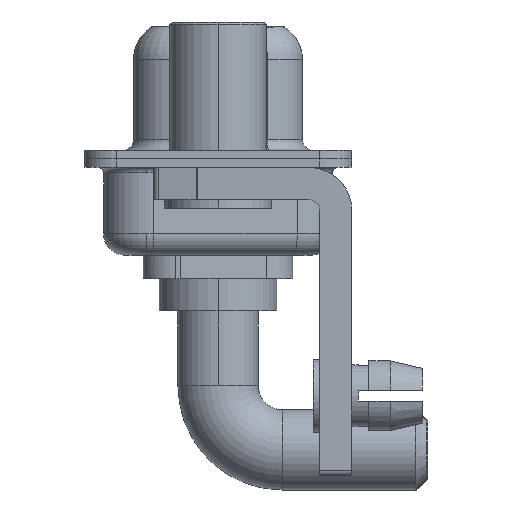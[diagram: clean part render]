
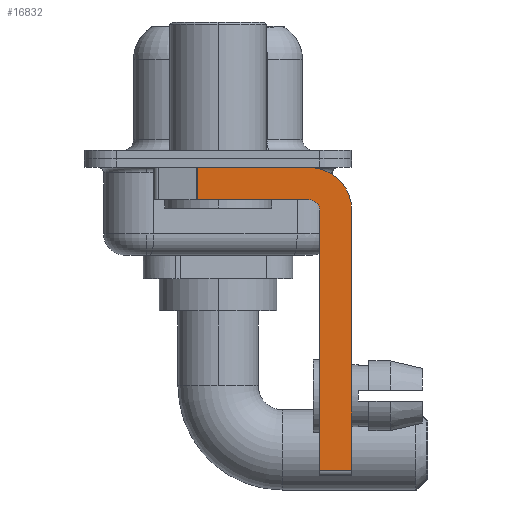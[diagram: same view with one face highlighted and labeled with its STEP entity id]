
A CAD part, left-side view. The second image highlights one B-rep face of the part: STEP entity #16832.
In plain terms, the highlighted planar face has unit normal (-1, 0, 0).
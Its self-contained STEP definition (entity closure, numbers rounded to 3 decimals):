
#1 = CARTESIAN_POINT ( 'NONE',  ( -2.9, -4.25, -1.9 ) ) ;
#162 = DIRECTION ( 'NONE',  ( 1., 0., 0. ) ) ;
#366 = AXIS2_PLACEMENT_3D ( 'NONE', #9549, #162, #2883 ) ;
#743 = ORIENTED_EDGE ( 'NONE', *, *, #10073, .F. ) ;
#809 = AXIS2_PLACEMENT_3D ( 'NONE', #10354, #12896, #15712 ) ;
#1100 = DIRECTION ( 'NONE',  ( 0., -1., 0. ) ) ;
#1345 = CARTESIAN_POINT ( 'NONE',  ( -2.9, 0.978, -1.9 ) ) ;
#1350 = VERTEX_POINT ( 'NONE', #8214 ) ;
#1498 = CARTESIAN_POINT ( 'NONE',  ( -2.9, -4.75, -14.55 ) ) ;
#1647 = ORIENTED_EDGE ( 'NONE', *, *, #7252, .F. ) ;
#1827 = PLANE ( 'NONE',  #366 ) ;
#1841 = DIRECTION ( 'NONE',  ( 0., 0., 1. ) ) ;
#2256 = DIRECTION ( 'NONE',  ( 0., 0., -1. ) ) ;
#2346 = EDGE_CURVE ( 'NONE', #8330, #3171, #4071, .T. ) ;
#2705 = CARTESIAN_POINT ( 'NONE',  ( -2.9, -6.25, -2.4 ) ) ;
#2883 = DIRECTION ( 'NONE',  ( 0., 0., -1. ) ) ;
#2997 = CARTESIAN_POINT ( 'NONE',  ( -2.9, -4.75, -2.4 ) ) ;
#3171 = VERTEX_POINT ( 'NONE', #12413 ) ;
#3783 = LINE ( 'NONE', #11503, #14538 ) ;
#4048 = CARTESIAN_POINT ( 'NONE',  ( -2.9, -6.25, -14.55 ) ) ;
#4071 = LINE ( 'NONE', #1345, #7500 ) ;
#4145 = VECTOR ( 'NONE', #15339, 1000. ) ;
#4991 = DIRECTION ( 'NONE',  ( 0., 0., 1. ) ) ;
#5455 = CIRCLE ( 'NONE', #7958, 0.5 ) ;
#5770 = CARTESIAN_POINT ( 'NONE',  ( -2.9, -4.75, -14.8 ) ) ;
#6132 = CIRCLE ( 'NONE', #809, 2. ) ;
#6222 = EDGE_CURVE ( 'NONE', #14532, #13422, #5455, .T. ) ;
#6990 = EDGE_LOOP ( 'NONE', ( #12298, #10099, #743, #17229, #1647, #15953, #10006, #7535 ) ) ;
#7252 = EDGE_CURVE ( 'NONE', #14864, #14532, #8662, .T. ) ;
#7500 = VECTOR ( 'NONE', #12145, 1000. ) ;
#7535 = ORIENTED_EDGE ( 'NONE', *, *, #10084, .F. ) ;
#7752 = LINE ( 'NONE', #11632, #12132 ) ;
#7958 = AXIS2_PLACEMENT_3D ( 'NONE', #11650, #16993, #4991 ) ;
#8214 = CARTESIAN_POINT ( 'NONE',  ( -2.9, -4.25, -0.4 ) ) ;
#8330 = VERTEX_POINT ( 'NONE', #16807 ) ;
#8662 = LINE ( 'NONE', #5770, #15976 ) ;
#9024 = LINE ( 'NONE', #14377, #4145 ) ;
#9549 = CARTESIAN_POINT ( 'NONE',  ( -2.9, -4.25, -2.4 ) ) ;
#10006 = ORIENTED_EDGE ( 'NONE', *, *, #15042, .F. ) ;
#10073 = EDGE_CURVE ( 'NONE', #13422, #3171, #3783, .T. ) ;
#10084 = EDGE_CURVE ( 'NONE', #1350, #16722, #6132, .T. ) ;
#10099 = ORIENTED_EDGE ( 'NONE', *, *, #2346, .T. ) ;
#10142 = VERTEX_POINT ( 'NONE', #4048 ) ;
#10262 = DIRECTION ( 'NONE',  ( 0., 1., 0. ) ) ;
#10354 = CARTESIAN_POINT ( 'NONE',  ( -2.9, -4.25, -2.4 ) ) ;
#10576 = EDGE_CURVE ( 'NONE', #8330, #1350, #9024, .T. ) ;
#11503 = CARTESIAN_POINT ( 'NONE',  ( -2.9, -4.25, -1.9 ) ) ;
#11632 = CARTESIAN_POINT ( 'NONE',  ( -2.9, -6.25, -2.4 ) ) ;
#11650 = CARTESIAN_POINT ( 'NONE',  ( -2.9, -4.25, -2.4 ) ) ;
#12132 = VECTOR ( 'NONE', #2256, 1000. ) ;
#12145 = DIRECTION ( 'NONE',  ( 0., 0., -1. ) ) ;
#12298 = ORIENTED_EDGE ( 'NONE', *, *, #10576, .F. ) ;
#12413 = CARTESIAN_POINT ( 'NONE',  ( -2.9, 0.978, -1.9 ) ) ;
#12896 = DIRECTION ( 'NONE',  ( 1., 0., 0. ) ) ;
#13422 = VERTEX_POINT ( 'NONE', #1 ) ;
#13781 = VECTOR ( 'NONE', #1100, 1000. ) ;
#14377 = CARTESIAN_POINT ( 'NONE',  ( -2.9, 3., -0.4 ) ) ;
#14436 = LINE ( 'NONE', #17059, #13781 ) ;
#14532 = VERTEX_POINT ( 'NONE', #2997 ) ;
#14538 = VECTOR ( 'NONE', #10262, 1000. ) ;
#14864 = VERTEX_POINT ( 'NONE', #1498 ) ;
#14980 = FACE_OUTER_BOUND ( 'NONE', #6990, .T. ) ;
#15042 = EDGE_CURVE ( 'NONE', #16722, #10142, #7752, .T. ) ;
#15104 = EDGE_CURVE ( 'NONE', #14864, #10142, #14436, .T. ) ;
#15339 = DIRECTION ( 'NONE',  ( 0., -1., 0. ) ) ;
#15712 = DIRECTION ( 'NONE',  ( 0., 0., -1. ) ) ;
#15953 = ORIENTED_EDGE ( 'NONE', *, *, #15104, .T. ) ;
#15976 = VECTOR ( 'NONE', #1841, 1000. ) ;
#16722 = VERTEX_POINT ( 'NONE', #2705 ) ;
#16807 = CARTESIAN_POINT ( 'NONE',  ( -2.9, 0.978, -0.4 ) ) ;
#16832 = ADVANCED_FACE ( 'NONE', ( #14980 ), #1827, .F. ) ;
#16993 = DIRECTION ( 'NONE',  ( -1., 0., 0. ) ) ;
#17059 = CARTESIAN_POINT ( 'NONE',  ( -2.9, -4.25, -14.55 ) ) ;
#17229 = ORIENTED_EDGE ( 'NONE', *, *, #6222, .F. ) ;
